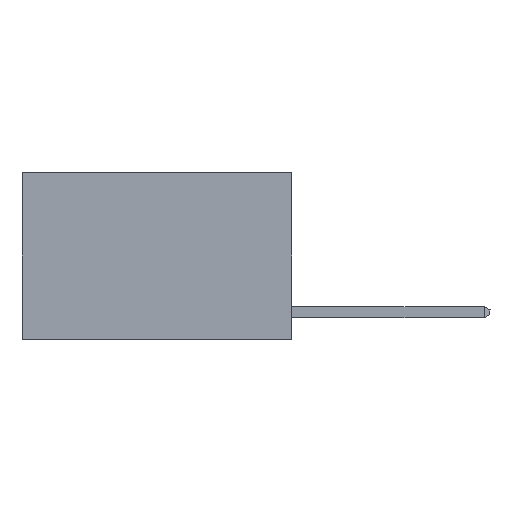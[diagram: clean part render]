
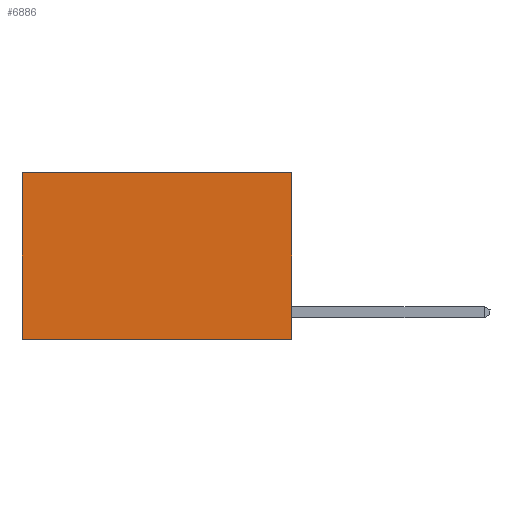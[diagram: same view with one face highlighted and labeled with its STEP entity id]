
A CAD part, left-side view. The second image highlights one B-rep face of the part: STEP entity #6886.
In plain terms, the highlighted planar face has unit normal (-1, 0, 0).
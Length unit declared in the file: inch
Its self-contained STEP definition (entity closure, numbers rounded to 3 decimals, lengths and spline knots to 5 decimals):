
#573 = CARTESIAN_POINT ( 'NONE',  ( 0.2625, 0.6, 0. ) ) ;
#1032 = DIRECTION ( 'NONE',  ( 1., 0., 0. ) ) ;
#1313 = LINE ( 'NONE', #7401, #17193 ) ;
#3643 = VERTEX_POINT ( 'NONE', #13313 ) ;
#4771 = VECTOR ( 'NONE', #17977, 39.37008 ) ;
#6780 = DIRECTION ( 'NONE',  ( 0., 1., 0. ) ) ;
#6886 = ADVANCED_FACE ( 'NONE', ( #17075 ), #19441, .F. ) ;
#7194 = DIRECTION ( 'NONE',  ( 0., 0., -1. ) ) ;
#7401 = CARTESIAN_POINT ( 'NONE',  ( 0.2625, 0.6, 0. ) ) ;
#8843 = AXIS2_PLACEMENT_3D ( 'NONE', #17989, #1032, #10554 ) ;
#8855 = VERTEX_POINT ( 'NONE', #18763 ) ;
#9550 = LINE ( 'NONE', #11459, #17280 ) ;
#9821 = EDGE_CURVE ( 'NONE', #3643, #8855, #13547, .T. ) ;
#10412 = CARTESIAN_POINT ( 'NONE',  ( 0.2625, 0., 0. ) ) ;
#10554 = DIRECTION ( 'NONE',  ( 0., 0., -1. ) ) ;
#11428 = VERTEX_POINT ( 'NONE', #14694 ) ;
#11459 = CARTESIAN_POINT ( 'NONE',  ( 0.2625, 0., 0. ) ) ;
#12152 = ORIENTED_EDGE ( 'NONE', *, *, #13452, .F. ) ;
#13313 = CARTESIAN_POINT ( 'NONE',  ( 0.2625, 0., 0. ) ) ;
#13452 = EDGE_CURVE ( 'NONE', #8855, #11428, #14084, .T. ) ;
#13547 = LINE ( 'NONE', #10412, #4771 ) ;
#13733 = EDGE_CURVE ( 'NONE', #15294, #11428, #1313, .T. ) ;
#14084 = LINE ( 'NONE', #16993, #19609 ) ;
#14433 = ORIENTED_EDGE ( 'NONE', *, *, #9821, .F. ) ;
#14694 = CARTESIAN_POINT ( 'NONE',  ( 0.2625, 0.6, -0.37 ) ) ;
#15159 = EDGE_LOOP ( 'NONE', ( #18219, #12152, #14433, #18884 ) ) ;
#15294 = VERTEX_POINT ( 'NONE', #573 ) ;
#16993 = CARTESIAN_POINT ( 'NONE',  ( 0.2625, 0., -0.37 ) ) ;
#17075 = FACE_OUTER_BOUND ( 'NONE', #15159, .T. ) ;
#17193 = VECTOR ( 'NONE', #7194, 39.37008 ) ;
#17280 = VECTOR ( 'NONE', #18955, 39.37008 ) ;
#17977 = DIRECTION ( 'NONE',  ( 0., 0., -1. ) ) ;
#17989 = CARTESIAN_POINT ( 'NONE',  ( 0.2625, 0., 0. ) ) ;
#18219 = ORIENTED_EDGE ( 'NONE', *, *, #13733, .T. ) ;
#18763 = CARTESIAN_POINT ( 'NONE',  ( 0.2625, 0., -0.37 ) ) ;
#18884 = ORIENTED_EDGE ( 'NONE', *, *, #19426, .T. ) ;
#18955 = DIRECTION ( 'NONE',  ( 0., 1., 0. ) ) ;
#19426 = EDGE_CURVE ( 'NONE', #3643, #15294, #9550, .T. ) ;
#19441 = PLANE ( 'NONE',  #8843 ) ;
#19609 = VECTOR ( 'NONE', #6780, 39.37008 ) ;
